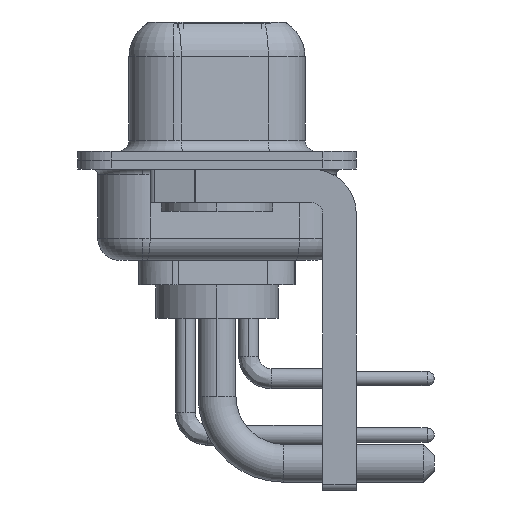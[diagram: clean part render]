
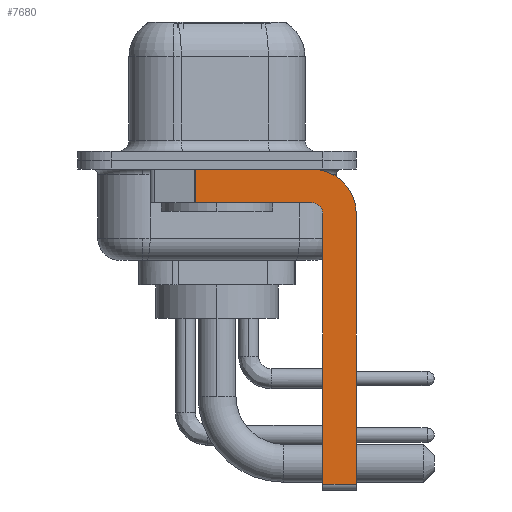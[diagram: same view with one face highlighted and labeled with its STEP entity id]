
A CAD part, left-side view. The second image highlights one B-rep face of the part: STEP entity #7680.
In plain terms, the highlighted planar face has unit normal (-1, 0, 0).
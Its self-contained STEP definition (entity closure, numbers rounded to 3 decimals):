
#141 = ORIENTED_EDGE ( 'NONE', *, *, #3231, .F. ) ;
#328 = EDGE_CURVE ( 'NONE', #13935, #5001, #12077, .T. ) ;
#664 = VECTOR ( 'NONE', #13891, 1000. ) ;
#1661 = CARTESIAN_POINT ( 'NONE',  ( -2.9, -4.25, -1.9 ) ) ;
#1795 = VECTOR ( 'NONE', #14642, 1000. ) ;
#2032 = EDGE_CURVE ( 'NONE', #15064, #17505, #14815, .T. ) ;
#2058 = AXIS2_PLACEMENT_3D ( 'NONE', #6640, #4958, #12582 ) ;
#2429 = DIRECTION ( 'NONE',  ( 0., 0., 1. ) ) ;
#2861 = LINE ( 'NONE', #8545, #1795 ) ;
#3231 = EDGE_CURVE ( 'NONE', #15064, #3472, #10434, .T. ) ;
#3472 = VERTEX_POINT ( 'NONE', #15482 ) ;
#3544 = CARTESIAN_POINT ( 'NONE',  ( -2.9, -4.75, -14.55 ) ) ;
#4350 = VECTOR ( 'NONE', #6050, 1000. ) ;
#4958 = DIRECTION ( 'NONE',  ( 1., 0., 0. ) ) ;
#5001 = VERTEX_POINT ( 'NONE', #12311 ) ;
#5248 = EDGE_LOOP ( 'NONE', ( #141, #11543, #24220, #14514, #11168, #13084, #5692, #20403 ) ) ;
#5376 = CARTESIAN_POINT ( 'NONE',  ( -2.9, -6.25, -2.4 ) ) ;
#5692 = ORIENTED_EDGE ( 'NONE', *, *, #23810, .F. ) ;
#6050 = DIRECTION ( 'NONE',  ( 0., -1., 0. ) ) ;
#6640 = CARTESIAN_POINT ( 'NONE',  ( -2.9, -4.25, -2.4 ) ) ;
#6716 = DIRECTION ( 'NONE',  ( -1., 0., 0. ) ) ;
#6936 = CARTESIAN_POINT ( 'NONE',  ( -2.9, -4.75, -14.8 ) ) ;
#7215 = FACE_OUTER_BOUND ( 'NONE', #5248, .T. ) ;
#7295 = CARTESIAN_POINT ( 'NONE',  ( -2.9, 0.978, -1.9 ) ) ;
#7419 = AXIS2_PLACEMENT_3D ( 'NONE', #21307, #9526, #21188 ) ;
#7680 = ADVANCED_FACE ( 'NONE', ( #7215 ), #23360, .F. ) ;
#8498 = EDGE_CURVE ( 'NONE', #3472, #13953, #23934, .T. ) ;
#8545 = CARTESIAN_POINT ( 'NONE',  ( -2.9, -6.25, -2.4 ) ) ;
#9526 = DIRECTION ( 'NONE',  ( 1., 0., 0. ) ) ;
#10126 = LINE ( 'NONE', #13658, #664 ) ;
#10434 = LINE ( 'NONE', #16258, #4350 ) ;
#11168 = ORIENTED_EDGE ( 'NONE', *, *, #16131, .F. ) ;
#11223 = CARTESIAN_POINT ( 'NONE',  ( -2.9, -4.75, -2.4 ) ) ;
#11543 = ORIENTED_EDGE ( 'NONE', *, *, #2032, .T. ) ;
#12077 = LINE ( 'NONE', #16223, #19881 ) ;
#12311 = CARTESIAN_POINT ( 'NONE',  ( -2.9, -6.25, -14.55 ) ) ;
#12582 = DIRECTION ( 'NONE',  ( 0., 0., -1. ) ) ;
#12900 = VERTEX_POINT ( 'NONE', #1661 ) ;
#13084 = ORIENTED_EDGE ( 'NONE', *, *, #328, .T. ) ;
#13528 = VECTOR ( 'NONE', #17648, 1000. ) ;
#13658 = CARTESIAN_POINT ( 'NONE',  ( -2.9, -4.25, -1.9 ) ) ;
#13718 = VECTOR ( 'NONE', #17266, 1000. ) ;
#13891 = DIRECTION ( 'NONE',  ( 0., 1., 0. ) ) ;
#13935 = VERTEX_POINT ( 'NONE', #3544 ) ;
#13953 = VERTEX_POINT ( 'NONE', #5376 ) ;
#14422 = DIRECTION ( 'NONE',  ( 0., -1., 0. ) ) ;
#14514 = ORIENTED_EDGE ( 'NONE', *, *, #22910, .F. ) ;
#14642 = DIRECTION ( 'NONE',  ( 0., 0., -1. ) ) ;
#14815 = LINE ( 'NONE', #7295, #13718 ) ;
#15011 = AXIS2_PLACEMENT_3D ( 'NONE', #24546, #6716, #2429 ) ;
#15064 = VERTEX_POINT ( 'NONE', #20085 ) ;
#15482 = CARTESIAN_POINT ( 'NONE',  ( -2.9, -4.25, -0.4 ) ) ;
#16131 = EDGE_CURVE ( 'NONE', #13935, #20356, #24634, .T. ) ;
#16223 = CARTESIAN_POINT ( 'NONE',  ( -2.9, -4.25, -14.55 ) ) ;
#16258 = CARTESIAN_POINT ( 'NONE',  ( -2.9, 3., -0.4 ) ) ;
#16414 = CARTESIAN_POINT ( 'NONE',  ( -2.9, 0.978, -1.9 ) ) ;
#17266 = DIRECTION ( 'NONE',  ( 0., 0., -1. ) ) ;
#17505 = VERTEX_POINT ( 'NONE', #16414 ) ;
#17648 = DIRECTION ( 'NONE',  ( 0., 0., 1. ) ) ;
#19881 = VECTOR ( 'NONE', #14422, 1000. ) ;
#19941 = CIRCLE ( 'NONE', #15011, 0.5 ) ;
#20085 = CARTESIAN_POINT ( 'NONE',  ( -2.9, 0.978, -0.4 ) ) ;
#20356 = VERTEX_POINT ( 'NONE', #11223 ) ;
#20403 = ORIENTED_EDGE ( 'NONE', *, *, #8498, .F. ) ;
#21188 = DIRECTION ( 'NONE',  ( 0., 0., -1. ) ) ;
#21307 = CARTESIAN_POINT ( 'NONE',  ( -2.9, -4.25, -2.4 ) ) ;
#22910 = EDGE_CURVE ( 'NONE', #20356, #12900, #19941, .T. ) ;
#23360 = PLANE ( 'NONE',  #7419 ) ;
#23810 = EDGE_CURVE ( 'NONE', #13953, #5001, #2861, .T. ) ;
#23934 = CIRCLE ( 'NONE', #2058, 2. ) ;
#24220 = ORIENTED_EDGE ( 'NONE', *, *, #24971, .F. ) ;
#24546 = CARTESIAN_POINT ( 'NONE',  ( -2.9, -4.25, -2.4 ) ) ;
#24634 = LINE ( 'NONE', #6936, #13528 ) ;
#24971 = EDGE_CURVE ( 'NONE', #12900, #17505, #10126, .T. ) ;
